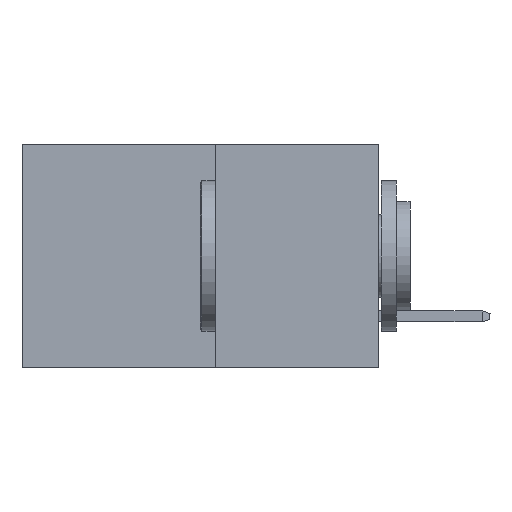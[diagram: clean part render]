
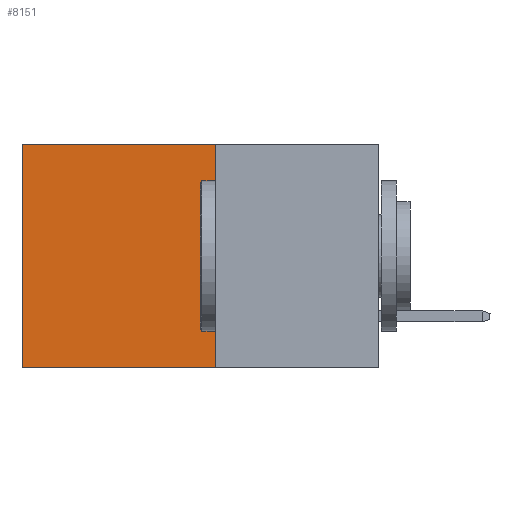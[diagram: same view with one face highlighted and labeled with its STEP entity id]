
A CAD part, left-side view. The second image highlights one B-rep face of the part: STEP entity #8151.
In plain terms, the highlighted planar face has unit normal (-1, 0, 0).
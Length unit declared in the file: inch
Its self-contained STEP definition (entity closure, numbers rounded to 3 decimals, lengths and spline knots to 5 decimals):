
#511 = ORIENTED_EDGE ( 'NONE', *, *, #6635, .F. ) ;
#932 = LINE ( 'NONE', #12963, #28914 ) ;
#2523 = EDGE_CURVE ( 'NONE', #22748, #17380, #28947, .T. ) ;
#4238 = ORIENTED_EDGE ( 'NONE', *, *, #14808, .F. ) ;
#4259 = VECTOR ( 'NONE', #25147, 39.37008 ) ;
#4943 = EDGE_CURVE ( 'NONE', #17380, #15710, #8905, .T. ) ;
#6062 = EDGE_LOOP ( 'NONE', ( #30539, #511, #4238, #17890 ) ) ;
#6635 = EDGE_CURVE ( 'NONE', #27798, #15710, #17237, .T. ) ;
#8007 = CARTESIAN_POINT ( 'NONE',  ( 0.277, 0.27, 0. ) ) ;
#8151 = ADVANCED_FACE ( 'NONE', ( #11155 ), #10329, .F. ) ;
#8905 = LINE ( 'NONE', #24158, #27570 ) ;
#9016 = CARTESIAN_POINT ( 'NONE',  ( 0.277, 0.27, -0.37 ) ) ;
#10329 = PLANE ( 'NONE',  #18453 ) ;
#11155 = FACE_OUTER_BOUND ( 'NONE', #6062, .T. ) ;
#12963 = CARTESIAN_POINT ( 'NONE',  ( 0.277, 0.27, -0.37 ) ) ;
#12991 = DIRECTION ( 'NONE',  ( 0., 0., -1. ) ) ;
#14808 = EDGE_CURVE ( 'NONE', #22748, #27798, #932, .T. ) ;
#15551 = VECTOR ( 'NONE', #24434, 39.37008 ) ;
#15582 = CARTESIAN_POINT ( 'NONE',  ( 0.277, 0.27, -0.37 ) ) ;
#15710 = VERTEX_POINT ( 'NONE', #26351 ) ;
#17237 = LINE ( 'NONE', #9016, #4259 ) ;
#17380 = VERTEX_POINT ( 'NONE', #25347 ) ;
#17890 = ORIENTED_EDGE ( 'NONE', *, *, #2523, .T. ) ;
#18453 = AXIS2_PLACEMENT_3D ( 'NONE', #19887, #20630, #20595 ) ;
#19887 = CARTESIAN_POINT ( 'NONE',  ( 0.277, 0.27, -0.37 ) ) ;
#20595 = DIRECTION ( 'NONE',  ( 0., 0., -1. ) ) ;
#20630 = DIRECTION ( 'NONE',  ( 1., 0., 0. ) ) ;
#22748 = VERTEX_POINT ( 'NONE', #32865 ) ;
#24158 = CARTESIAN_POINT ( 'NONE',  ( 0.277, 0.59, -0.37 ) ) ;
#24262 = DIRECTION ( 'NONE',  ( 0., 0., -1. ) ) ;
#24434 = DIRECTION ( 'NONE',  ( 0., 1., 0. ) ) ;
#25147 = DIRECTION ( 'NONE',  ( 0., 1., 0. ) ) ;
#25347 = CARTESIAN_POINT ( 'NONE',  ( 0.277, 0.59, 0. ) ) ;
#26351 = CARTESIAN_POINT ( 'NONE',  ( 0.277, 0.59, -0.37 ) ) ;
#27570 = VECTOR ( 'NONE', #24262, 39.37008 ) ;
#27798 = VERTEX_POINT ( 'NONE', #15582 ) ;
#28914 = VECTOR ( 'NONE', #12991, 39.37008 ) ;
#28947 = LINE ( 'NONE', #8007, #15551 ) ;
#30539 = ORIENTED_EDGE ( 'NONE', *, *, #4943, .T. ) ;
#32865 = CARTESIAN_POINT ( 'NONE',  ( 0.277, 0.27, 0. ) ) ;
